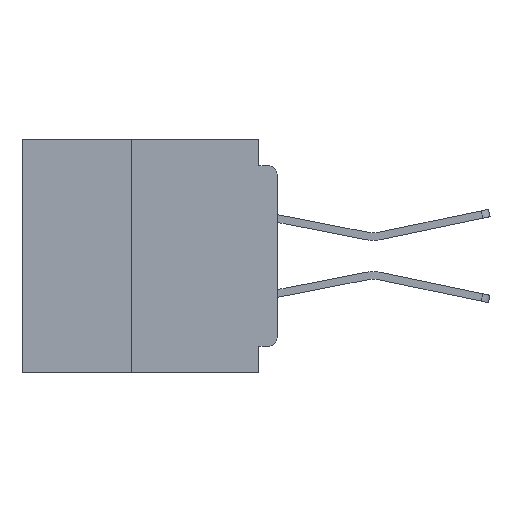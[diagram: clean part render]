
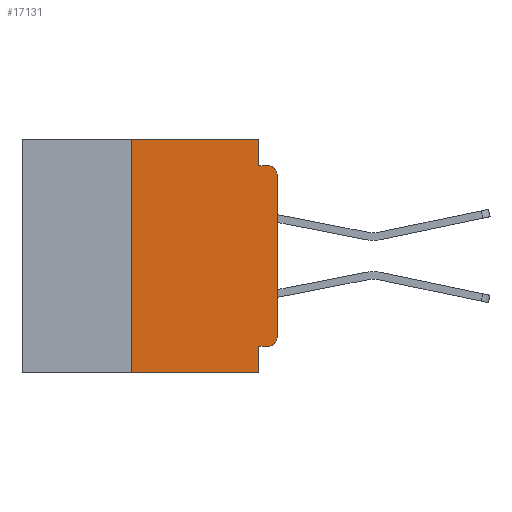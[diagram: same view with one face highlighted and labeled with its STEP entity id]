
A CAD part, left-side view. The second image highlights one B-rep face of the part: STEP entity #17131.
In plain terms, the highlighted planar face has unit normal (-1, 0, 0).
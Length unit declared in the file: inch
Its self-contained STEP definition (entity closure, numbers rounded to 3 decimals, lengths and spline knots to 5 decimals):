
#1107 = CARTESIAN_POINT ( 'NONE',  ( 0., 0.015, -0.06 ) ) ;
#1135 = EDGE_CURVE ( 'NONE', #10322, #16659, #43215, .T. ) ;
#2566 = VECTOR ( 'NONE', #15593, 39.37008 ) ;
#3594 = CARTESIAN_POINT ( 'NONE',  ( 0., 0.25, -0.4 ) ) ;
#3820 = EDGE_CURVE ( 'NONE', #4427, #4624, #11659, .T. ) ;
#4131 = VECTOR ( 'NONE', #13278, 39.37008 ) ;
#4283 = CARTESIAN_POINT ( 'NONE',  ( 0., 0.015, -0.355 ) ) ;
#4427 = VERTEX_POINT ( 'NONE', #24362 ) ;
#4562 = DIRECTION ( 'NONE',  ( 0., 0., -1. ) ) ;
#4624 = VERTEX_POINT ( 'NONE', #25231 ) ;
#4648 = CARTESIAN_POINT ( 'NONE',  ( 0., 0.015, -0.045 ) ) ;
#5873 = CARTESIAN_POINT ( 'NONE',  ( 0., 0.437, 0. ) ) ;
#6478 = LINE ( 'NONE', #17459, #14418 ) ;
#7632 = ORIENTED_EDGE ( 'NONE', *, *, #17735, .T. ) ;
#7822 = ORIENTED_EDGE ( 'NONE', *, *, #23926, .T. ) ;
#8372 = CARTESIAN_POINT ( 'NONE',  ( 0., 0.031, -0.4 ) ) ;
#8688 = AXIS2_PLACEMENT_3D ( 'NONE', #1107, #24758, #4562 ) ;
#8707 = ORIENTED_EDGE ( 'NONE', *, *, #40630, .F. ) ;
#8824 = CARTESIAN_POINT ( 'NONE',  ( 0., 0.437, -0.4 ) ) ;
#8934 = CARTESIAN_POINT ( 'NONE',  ( 0., 0.031, -0.045 ) ) ;
#9330 = DIRECTION ( 'NONE',  ( 0., 0., -1. ) ) ;
#10005 = LINE ( 'NONE', #15080, #34689 ) ;
#10322 = VERTEX_POINT ( 'NONE', #4283 ) ;
#11659 = LINE ( 'NONE', #8824, #2566 ) ;
#11863 = DIRECTION ( 'NONE',  ( 0., -1., 0. ) ) ;
#12558 = PLANE ( 'NONE',  #32350 ) ;
#12898 = CARTESIAN_POINT ( 'NONE',  ( 0., 0.25, 0. ) ) ;
#13169 = LINE ( 'NONE', #20017, #4131 ) ;
#13278 = DIRECTION ( 'NONE',  ( 0., 0., -1. ) ) ;
#13348 = VERTEX_POINT ( 'NONE', #37222 ) ;
#14418 = VECTOR ( 'NONE', #40829, 39.37008 ) ;
#15080 = CARTESIAN_POINT ( 'NONE',  ( 0., 0., -0.045 ) ) ;
#15593 = DIRECTION ( 'NONE',  ( 0., -1., 0. ) ) ;
#15740 = DIRECTION ( 'NONE',  ( 0., 0., 1. ) ) ;
#16515 = ORIENTED_EDGE ( 'NONE', *, *, #24014, .F. ) ;
#16659 = VERTEX_POINT ( 'NONE', #33102 ) ;
#17131 = ADVANCED_FACE ( 'NONE', ( #28764 ), #12558, .F. ) ;
#17459 = CARTESIAN_POINT ( 'NONE',  ( 0., 0.437, 0. ) ) ;
#17735 = EDGE_CURVE ( 'NONE', #16659, #27233, #21913, .T. ) ;
#17756 = LINE ( 'NONE', #8372, #18803 ) ;
#18348 = VECTOR ( 'NONE', #20762, 39.37008 ) ;
#18803 = VECTOR ( 'NONE', #35085, 39.37008 ) ;
#19636 = EDGE_LOOP ( 'NONE', ( #7632, #7822, #16515, #43007, #8707, #37233, #24552, #27541, #42155, #23878 ) ) ;
#20017 = CARTESIAN_POINT ( 'NONE',  ( 0., 0.031, 0. ) ) ;
#20616 = VERTEX_POINT ( 'NONE', #8934 ) ;
#20762 = DIRECTION ( 'NONE',  ( 0., 1., 0. ) ) ;
#21489 = EDGE_CURVE ( 'NONE', #13348, #20616, #13169, .T. ) ;
#21594 = VECTOR ( 'NONE', #23818, 39.37008 ) ;
#21774 = VERTEX_POINT ( 'NONE', #4648 ) ;
#21913 = LINE ( 'NONE', #35818, #40181 ) ;
#23818 = DIRECTION ( 'NONE',  ( 0., 0., 1. ) ) ;
#23878 = ORIENTED_EDGE ( 'NONE', *, *, #1135, .T. ) ;
#23926 = EDGE_CURVE ( 'NONE', #27233, #21774, #29976, .T. ) ;
#24014 = EDGE_CURVE ( 'NONE', #20616, #21774, #10005, .T. ) ;
#24362 = CARTESIAN_POINT ( 'NONE',  ( 0., 0.25, -0.4 ) ) ;
#24385 = EDGE_CURVE ( 'NONE', #4427, #32174, #30528, .T. ) ;
#24552 = ORIENTED_EDGE ( 'NONE', *, *, #3820, .T. ) ;
#24758 = DIRECTION ( 'NONE',  ( -1., 0., 0. ) ) ;
#25231 = CARTESIAN_POINT ( 'NONE',  ( 0., 0.031, -0.4 ) ) ;
#25772 = EDGE_CURVE ( 'NONE', #10322, #41614, #37216, .T. ) ;
#26097 = CARTESIAN_POINT ( 'NONE',  ( 0., 0., -0.06 ) ) ;
#27233 = VERTEX_POINT ( 'NONE', #26097 ) ;
#27518 = CARTESIAN_POINT ( 'NONE',  ( 0., 0., -0.355 ) ) ;
#27541 = ORIENTED_EDGE ( 'NONE', *, *, #38892, .F. ) ;
#28764 = FACE_OUTER_BOUND ( 'NONE', #19636, .T. ) ;
#29441 = DIRECTION ( 'NONE',  ( 1., 0., 0. ) ) ;
#29976 = CIRCLE ( 'NONE', #8688, 0.015 ) ;
#30528 = LINE ( 'NONE', #3594, #21594 ) ;
#32174 = VERTEX_POINT ( 'NONE', #12898 ) ;
#32350 = AXIS2_PLACEMENT_3D ( 'NONE', #5873, #29441, #9330 ) ;
#32599 = CARTESIAN_POINT ( 'NONE',  ( 0., 0.031, -0.355 ) ) ;
#33102 = CARTESIAN_POINT ( 'NONE',  ( 0., 0., -0.34 ) ) ;
#34689 = VECTOR ( 'NONE', #11863, 39.37008 ) ;
#35085 = DIRECTION ( 'NONE',  ( 0., 0., -1. ) ) ;
#35818 = CARTESIAN_POINT ( 'NONE',  ( 0., 0., 0. ) ) ;
#37216 = LINE ( 'NONE', #27518, #18348 ) ;
#37222 = CARTESIAN_POINT ( 'NONE',  ( 0., 0.031, 0. ) ) ;
#37233 = ORIENTED_EDGE ( 'NONE', *, *, #24385, .F. ) ;
#38458 = AXIS2_PLACEMENT_3D ( 'NONE', #38705, #38657, #38559 ) ;
#38559 = DIRECTION ( 'NONE',  ( 0., 0., -1. ) ) ;
#38657 = DIRECTION ( 'NONE',  ( -1., 0., 0. ) ) ;
#38705 = CARTESIAN_POINT ( 'NONE',  ( 0., 0.015, -0.34 ) ) ;
#38892 = EDGE_CURVE ( 'NONE', #41614, #4624, #17756, .T. ) ;
#40181 = VECTOR ( 'NONE', #15740, 39.37008 ) ;
#40630 = EDGE_CURVE ( 'NONE', #32174, #13348, #6478, .T. ) ;
#40829 = DIRECTION ( 'NONE',  ( 0., -1., 0. ) ) ;
#41614 = VERTEX_POINT ( 'NONE', #32599 ) ;
#42155 = ORIENTED_EDGE ( 'NONE', *, *, #25772, .F. ) ;
#43007 = ORIENTED_EDGE ( 'NONE', *, *, #21489, .F. ) ;
#43215 = CIRCLE ( 'NONE', #38458, 0.015 ) ;
